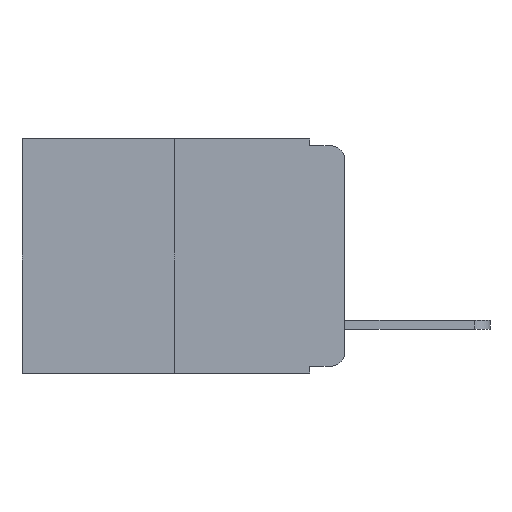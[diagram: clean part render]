
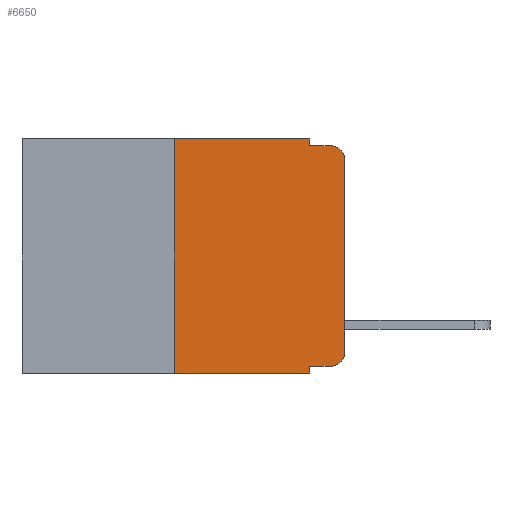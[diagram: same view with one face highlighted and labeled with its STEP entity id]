
A CAD part, left-side view. The second image highlights one B-rep face of the part: STEP entity #6650.
In plain terms, the highlighted planar face has unit normal (-1, 0, 0).
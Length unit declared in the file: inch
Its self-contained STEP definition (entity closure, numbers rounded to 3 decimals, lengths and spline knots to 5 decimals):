
#8 = ORIENTED_EDGE ( 'NONE', *, *, #5938, .F. ) ;
#331 = DIRECTION ( 'NONE',  ( 0., 0., -1. ) ) ;
#738 = PLANE ( 'NONE',  #8309 ) ;
#1042 = CARTESIAN_POINT ( 'NONE',  ( 0., 0.473, 0. ) ) ;
#1106 = DIRECTION ( 'NONE',  ( 0., 0., -1. ) ) ;
#1346 = ORIENTED_EDGE ( 'NONE', *, *, #7860, .F. ) ;
#1388 = DIRECTION ( 'NONE',  ( 0., 0., -1. ) ) ;
#1717 = CARTESIAN_POINT ( 'NONE',  ( 0., 0.051, -0.343 ) ) ;
#1846 = VERTEX_POINT ( 'NONE', #9464 ) ;
#2107 = EDGE_CURVE ( 'NONE', #4399, #4698, #5630, .T. ) ;
#2468 = VERTEX_POINT ( 'NONE', #4557 ) ;
#2870 = CARTESIAN_POINT ( 'NONE',  ( 0., 0.051, 0. ) ) ;
#3440 = CARTESIAN_POINT ( 'NONE',  ( 0., 0., -0.03 ) ) ;
#3483 = DIRECTION ( 'NONE',  ( 0., 0., 1. ) ) ;
#3509 = DIRECTION ( 'NONE',  ( 0., 0., -1. ) ) ;
#3876 = CARTESIAN_POINT ( 'NONE',  ( 0., 0.25, 0. ) ) ;
#3918 = EDGE_CURVE ( 'NONE', #7858, #15705, #11900, .T. ) ;
#4153 = ORIENTED_EDGE ( 'NONE', *, *, #5055, .T. ) ;
#4301 = AXIS2_PLACEMENT_3D ( 'NONE', #11081, #8625, #1106 ) ;
#4399 = VERTEX_POINT ( 'NONE', #6797 ) ;
#4483 = CARTESIAN_POINT ( 'NONE',  ( 0., 0.051, 0. ) ) ;
#4557 = CARTESIAN_POINT ( 'NONE',  ( 0., 0.25, -0.343 ) ) ;
#4652 = VECTOR ( 'NONE', #3509, 39.37008 ) ;
#4698 = VERTEX_POINT ( 'NONE', #3440 ) ;
#5055 = EDGE_CURVE ( 'NONE', #4698, #1846, #7491, .T. ) ;
#5299 = LINE ( 'NONE', #7065, #8352 ) ;
#5304 = EDGE_CURVE ( 'NONE', #15705, #4399, #12451, .T. ) ;
#5348 = ORIENTED_EDGE ( 'NONE', *, *, #2107, .T. ) ;
#5432 = LINE ( 'NONE', #13363, #4652 ) ;
#5557 = VERTEX_POINT ( 'NONE', #4483 ) ;
#5630 = LINE ( 'NONE', #7532, #14618 ) ;
#5720 = DIRECTION ( 'NONE',  ( 0., -1., 0. ) ) ;
#5756 = LINE ( 'NONE', #10770, #7291 ) ;
#5788 = DIRECTION ( 'NONE',  ( 0., -1., 0. ) ) ;
#5938 = EDGE_CURVE ( 'NONE', #7858, #11471, #6905, .T. ) ;
#6042 = VECTOR ( 'NONE', #10636, 39.37008 ) ;
#6115 = FACE_OUTER_BOUND ( 'NONE', #10249, .T. ) ;
#6534 = VECTOR ( 'NONE', #331, 39.37008 ) ;
#6650 = ADVANCED_FACE ( 'NONE', ( #6115 ), #738, .F. ) ;
#6797 = CARTESIAN_POINT ( 'NONE',  ( 0., 0., -0.313 ) ) ;
#6863 = CARTESIAN_POINT ( 'NONE',  ( 0., 0.473, 0. ) ) ;
#6905 = LINE ( 'NONE', #2870, #6534 ) ;
#7050 = ORIENTED_EDGE ( 'NONE', *, *, #12178, .T. ) ;
#7065 = CARTESIAN_POINT ( 'NONE',  ( 0., 0.051, -0.01 ) ) ;
#7291 = VECTOR ( 'NONE', #3483, 39.37008 ) ;
#7368 = EDGE_CURVE ( 'NONE', #8878, #5557, #14292, .T. ) ;
#7491 = CIRCLE ( 'NONE', #4301, 0.02 ) ;
#7532 = CARTESIAN_POINT ( 'NONE',  ( 0., 0., 0. ) ) ;
#7691 = VERTEX_POINT ( 'NONE', #10206 ) ;
#7858 = VERTEX_POINT ( 'NONE', #12125 ) ;
#7860 = EDGE_CURVE ( 'NONE', #7691, #1846, #5299, .T. ) ;
#7981 = DIRECTION ( 'NONE',  ( 0., 0., -1. ) ) ;
#8309 = AXIS2_PLACEMENT_3D ( 'NONE', #6863, #14240, #7981 ) ;
#8352 = VECTOR ( 'NONE', #10766, 39.37008 ) ;
#8625 = DIRECTION ( 'NONE',  ( -1., 0., 0. ) ) ;
#8736 = DIRECTION ( 'NONE',  ( -1., 0., 0. ) ) ;
#8754 = DIRECTION ( 'NONE',  ( 0., 0., 1. ) ) ;
#8878 = VERTEX_POINT ( 'NONE', #3876 ) ;
#9306 = AXIS2_PLACEMENT_3D ( 'NONE', #14827, #8736, #1388 ) ;
#9464 = CARTESIAN_POINT ( 'NONE',  ( 0., 0.02, -0.01 ) ) ;
#9964 = EDGE_CURVE ( 'NONE', #5557, #7691, #5432, .T. ) ;
#10206 = CARTESIAN_POINT ( 'NONE',  ( 0., 0.051, -0.01 ) ) ;
#10249 = EDGE_LOOP ( 'NONE', ( #5348, #4153, #1346, #12723, #11656, #15246, #7050, #8, #14931, #11736 ) ) ;
#10636 = DIRECTION ( 'NONE',  ( 0., -1., 0. ) ) ;
#10766 = DIRECTION ( 'NONE',  ( 0., -1., 0. ) ) ;
#10770 = CARTESIAN_POINT ( 'NONE',  ( 0., 0.25, 0. ) ) ;
#11081 = CARTESIAN_POINT ( 'NONE',  ( 0., 0.02, -0.03 ) ) ;
#11471 = VERTEX_POINT ( 'NONE', #1717 ) ;
#11656 = ORIENTED_EDGE ( 'NONE', *, *, #7368, .F. ) ;
#11736 = ORIENTED_EDGE ( 'NONE', *, *, #5304, .T. ) ;
#11900 = LINE ( 'NONE', #14112, #14366 ) ;
#11954 = CARTESIAN_POINT ( 'NONE',  ( 0., 0.473, -0.343 ) ) ;
#12125 = CARTESIAN_POINT ( 'NONE',  ( 0., 0.051, -0.333 ) ) ;
#12178 = EDGE_CURVE ( 'NONE', #2468, #11471, #15419, .T. ) ;
#12451 = CIRCLE ( 'NONE', #9306, 0.02 ) ;
#12723 = ORIENTED_EDGE ( 'NONE', *, *, #9964, .F. ) ;
#13363 = CARTESIAN_POINT ( 'NONE',  ( 0., 0.051, 0. ) ) ;
#13731 = VECTOR ( 'NONE', #5788, 39.37008 ) ;
#14112 = CARTESIAN_POINT ( 'NONE',  ( 0., 0.051, -0.333 ) ) ;
#14240 = DIRECTION ( 'NONE',  ( 1., 0., 0. ) ) ;
#14292 = LINE ( 'NONE', #1042, #13731 ) ;
#14366 = VECTOR ( 'NONE', #5720, 39.37008 ) ;
#14618 = VECTOR ( 'NONE', #8754, 39.37008 ) ;
#14722 = CARTESIAN_POINT ( 'NONE',  ( 0., 0.02, -0.333 ) ) ;
#14827 = CARTESIAN_POINT ( 'NONE',  ( 0., 0.02, -0.313 ) ) ;
#14931 = ORIENTED_EDGE ( 'NONE', *, *, #3918, .T. ) ;
#15246 = ORIENTED_EDGE ( 'NONE', *, *, #15523, .F. ) ;
#15419 = LINE ( 'NONE', #11954, #6042 ) ;
#15523 = EDGE_CURVE ( 'NONE', #2468, #8878, #5756, .T. ) ;
#15705 = VERTEX_POINT ( 'NONE', #14722 ) ;
